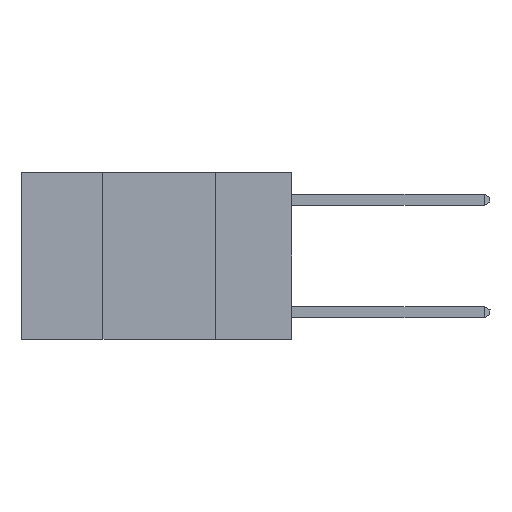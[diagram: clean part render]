
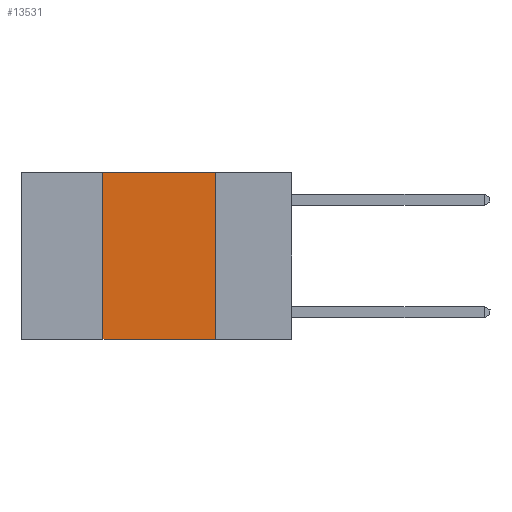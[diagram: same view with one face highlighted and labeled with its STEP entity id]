
A CAD part, left-side view. The second image highlights one B-rep face of the part: STEP entity #13531.
In plain terms, the highlighted planar face has unit normal (-1, 0, 0).
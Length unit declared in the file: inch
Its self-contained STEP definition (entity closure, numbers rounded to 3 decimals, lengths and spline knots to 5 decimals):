
#1089 = EDGE_CURVE ( 'NONE', #9941, #7375, #28044, .T. ) ;
#3960 = CARTESIAN_POINT ( 'NONE',  ( 0., 0.42, 0. ) ) ;
#3998 = CARTESIAN_POINT ( 'NONE',  ( 0., 0.17, 0. ) ) ;
#4450 = EDGE_LOOP ( 'NONE', ( #14725, #13398, #20797, #11303 ) ) ;
#6399 = LINE ( 'NONE', #3960, #12479 ) ;
#7375 = VERTEX_POINT ( 'NONE', #27951 ) ;
#9941 = VERTEX_POINT ( 'NONE', #3998 ) ;
#10468 = CARTESIAN_POINT ( 'NONE',  ( 0., 0.6, 0. ) ) ;
#11303 = ORIENTED_EDGE ( 'NONE', *, *, #15603, .T. ) ;
#11422 = CARTESIAN_POINT ( 'NONE',  ( 0., 0.6, -0.37 ) ) ;
#12479 = VECTOR ( 'NONE', #28729, 39.37008 ) ;
#12747 = DIRECTION ( 'NONE',  ( 1., 0., 0. ) ) ;
#13027 = VECTOR ( 'NONE', #20517, 39.37008 ) ;
#13398 = ORIENTED_EDGE ( 'NONE', *, *, #28033, .F. ) ;
#13531 = ADVANCED_FACE ( 'NONE', ( #23662 ), #17222, .F. ) ;
#14725 = ORIENTED_EDGE ( 'NONE', *, *, #1089, .F. ) ;
#14974 = VECTOR ( 'NONE', #24740, 39.37008 ) ;
#15177 = DIRECTION ( 'NONE',  ( 0., 0., -1. ) ) ;
#15603 = EDGE_CURVE ( 'NONE', #16924, #7375, #24961, .T. ) ;
#15752 = CARTESIAN_POINT ( 'NONE',  ( 0., 0.17, 0. ) ) ;
#16187 = VECTOR ( 'NONE', #15177, 39.37008 ) ;
#16924 = VERTEX_POINT ( 'NONE', #24923 ) ;
#17222 = PLANE ( 'NONE',  #17941 ) ;
#17941 = AXIS2_PLACEMENT_3D ( 'NONE', #10468, #12747, #28412 ) ;
#20517 = DIRECTION ( 'NONE',  ( 0., -1., 0. ) ) ;
#20797 = ORIENTED_EDGE ( 'NONE', *, *, #27916, .F. ) ;
#20921 = VERTEX_POINT ( 'NONE', #28966 ) ;
#20956 = LINE ( 'NONE', #29079, #14974 ) ;
#23662 = FACE_OUTER_BOUND ( 'NONE', #4450, .T. ) ;
#24740 = DIRECTION ( 'NONE',  ( 0., -1., 0. ) ) ;
#24923 = CARTESIAN_POINT ( 'NONE',  ( 0., 0.42, -0.37 ) ) ;
#24961 = LINE ( 'NONE', #11422, #13027 ) ;
#27916 = EDGE_CURVE ( 'NONE', #16924, #20921, #6399, .T. ) ;
#27951 = CARTESIAN_POINT ( 'NONE',  ( 0., 0.17, -0.37 ) ) ;
#28033 = EDGE_CURVE ( 'NONE', #20921, #9941, #20956, .T. ) ;
#28044 = LINE ( 'NONE', #15752, #16187 ) ;
#28412 = DIRECTION ( 'NONE',  ( 0., 0., -1. ) ) ;
#28729 = DIRECTION ( 'NONE',  ( 0., 0., 1. ) ) ;
#28966 = CARTESIAN_POINT ( 'NONE',  ( 0., 0.42, 0. ) ) ;
#29079 = CARTESIAN_POINT ( 'NONE',  ( 0., 0.6, 0. ) ) ;
